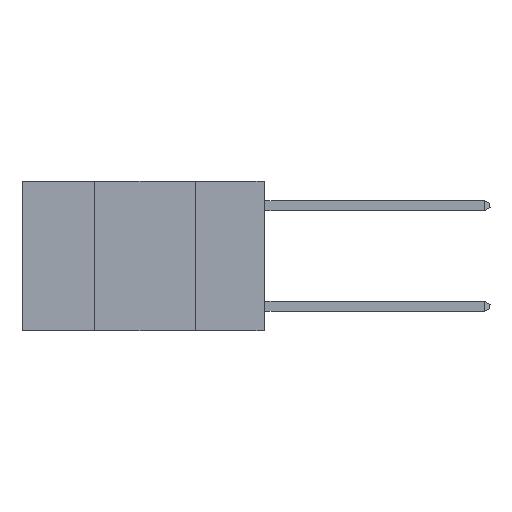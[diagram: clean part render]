
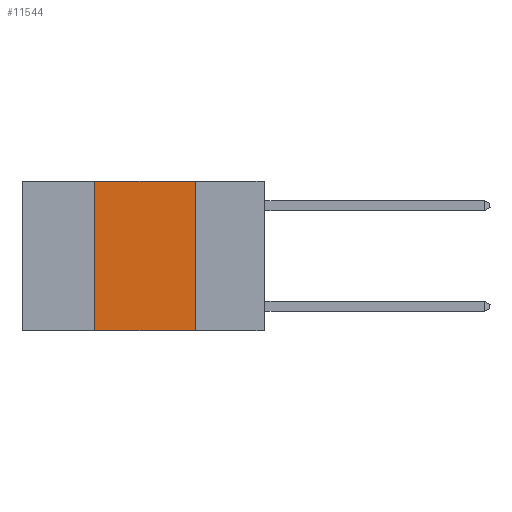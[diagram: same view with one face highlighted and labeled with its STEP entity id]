
A CAD part, left-side view. The second image highlights one B-rep face of the part: STEP entity #11544.
In plain terms, the highlighted planar face has unit normal (-1, 0, 0).
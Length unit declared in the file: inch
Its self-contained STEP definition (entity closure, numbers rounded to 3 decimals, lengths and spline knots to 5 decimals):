
#184 = VECTOR ( 'NONE', #4329, 39.37008 ) ;
#239 = CARTESIAN_POINT ( 'NONE',  ( 0., 0.6, -0.37 ) ) ;
#1286 = VERTEX_POINT ( 'NONE', #2834 ) ;
#1433 = ORIENTED_EDGE ( 'NONE', *, *, #3171, .T. ) ;
#1619 = VECTOR ( 'NONE', #7386, 39.37008 ) ;
#2303 = CARTESIAN_POINT ( 'NONE',  ( 0., 0.6, 0. ) ) ;
#2834 = CARTESIAN_POINT ( 'NONE',  ( 0., 0.17, 0. ) ) ;
#3171 = EDGE_CURVE ( 'NONE', #6530, #5797, #9764, .T. ) ;
#3245 = CARTESIAN_POINT ( 'NONE',  ( 0., 0.17, 0. ) ) ;
#3347 = CARTESIAN_POINT ( 'NONE',  ( 0., 0.17, -0.37 ) ) ;
#4055 = ORIENTED_EDGE ( 'NONE', *, *, #7486, .F. ) ;
#4329 = DIRECTION ( 'NONE',  ( 0., 0., 1. ) ) ;
#4390 = LINE ( 'NONE', #10776, #184 ) ;
#4600 = PLANE ( 'NONE',  #8221 ) ;
#4698 = EDGE_CURVE ( 'NONE', #1286, #5797, #6253, .T. ) ;
#5188 = CARTESIAN_POINT ( 'NONE',  ( 0., 0.6, 0. ) ) ;
#5409 = ORIENTED_EDGE ( 'NONE', *, *, #6399, .F. ) ;
#5797 = VERTEX_POINT ( 'NONE', #3347 ) ;
#5840 = ORIENTED_EDGE ( 'NONE', *, *, #4698, .F. ) ;
#6110 = VERTEX_POINT ( 'NONE', #13004 ) ;
#6253 = LINE ( 'NONE', #3245, #1619 ) ;
#6315 = LINE ( 'NONE', #5188, #7700 ) ;
#6399 = EDGE_CURVE ( 'NONE', #6110, #1286, #6315, .T. ) ;
#6530 = VERTEX_POINT ( 'NONE', #9560 ) ;
#6735 = DIRECTION ( 'NONE',  ( 0., -1., 0. ) ) ;
#7386 = DIRECTION ( 'NONE',  ( 0., 0., -1. ) ) ;
#7486 = EDGE_CURVE ( 'NONE', #6530, #6110, #4390, .T. ) ;
#7700 = VECTOR ( 'NONE', #10677, 39.37008 ) ;
#7863 = DIRECTION ( 'NONE',  ( 1., 0., 0. ) ) ;
#8221 = AXIS2_PLACEMENT_3D ( 'NONE', #2303, #7863, #11165 ) ;
#8624 = FACE_OUTER_BOUND ( 'NONE', #13740, .T. ) ;
#9560 = CARTESIAN_POINT ( 'NONE',  ( 0., 0.42, -0.37 ) ) ;
#9764 = LINE ( 'NONE', #239, #10464 ) ;
#10464 = VECTOR ( 'NONE', #6735, 39.37008 ) ;
#10677 = DIRECTION ( 'NONE',  ( 0., -1., 0. ) ) ;
#10776 = CARTESIAN_POINT ( 'NONE',  ( 0., 0.42, 0. ) ) ;
#11165 = DIRECTION ( 'NONE',  ( 0., 0., -1. ) ) ;
#11544 = ADVANCED_FACE ( 'NONE', ( #8624 ), #4600, .F. ) ;
#13004 = CARTESIAN_POINT ( 'NONE',  ( 0., 0.42, 0. ) ) ;
#13740 = EDGE_LOOP ( 'NONE', ( #5840, #5409, #4055, #1433 ) ) ;
